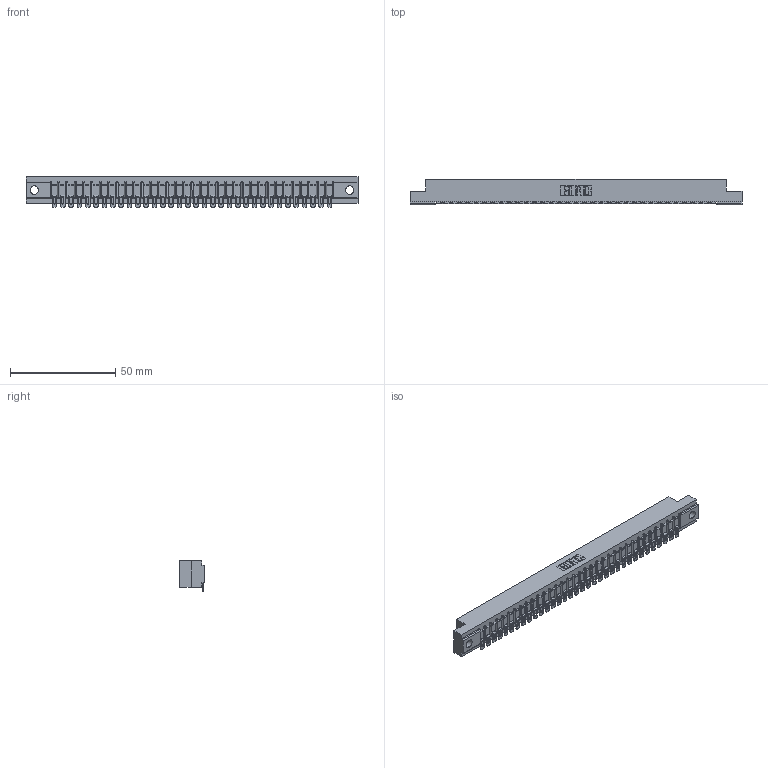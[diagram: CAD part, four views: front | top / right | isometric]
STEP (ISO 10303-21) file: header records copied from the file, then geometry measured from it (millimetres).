
FILE_DESCRIPTION (( 'STEP AP203' ), '1' );
FILE_NAME ('307-034-554-104.STEP', '2019-09-05T06:45:33', ( '' ), ( '' ), 'SwSTEP 2.0', 'SolidWorks 2016', '' );
FILE_SCHEMA (( 'CONFIG_CONTROL_DESIGN' ));
Length unit declared in the file: inch
Products named in the file (3): 307-034-554-104; 307 Part_.156 Dia Mounting Holes; 307-290-002_554
Assembly tree (35 placements, depth 2):
  307-034-554-104
    307 Part_.156 Dia Mounting Holes
    307-290-002_554  x34
Bounding box: 157.73 x 12.01 x 14.52 mm (x, y, z)
Volume: 16726.2 mm3; surface area: 20822.4 mm2
Topology: 35 solids, 35 shells, 2921 faces, 8961 edges, 5878 vertices
Faces by surface type: plane 1648, cylinder 1203, sphere 70
Entity records: 31517 total; most frequent: CARTESIAN_POINT 5320, ORIENTED_EDGE 5308, DIRECTION 5170, EDGE_CURVE 2654, VECTOR 2030, LINE 2030, VERTEX_POINT 1720, AXIS2_PLACEMENT_3D 1570
